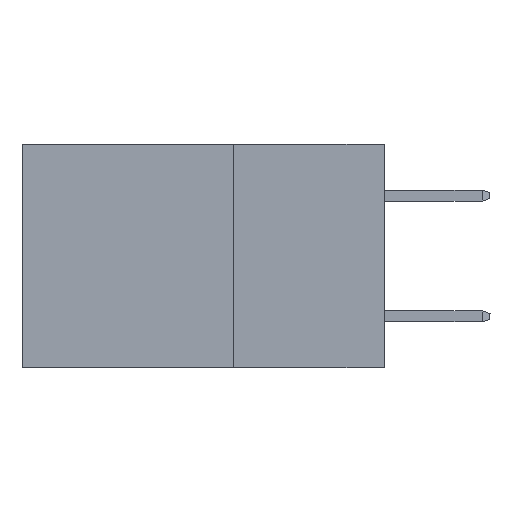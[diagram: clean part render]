
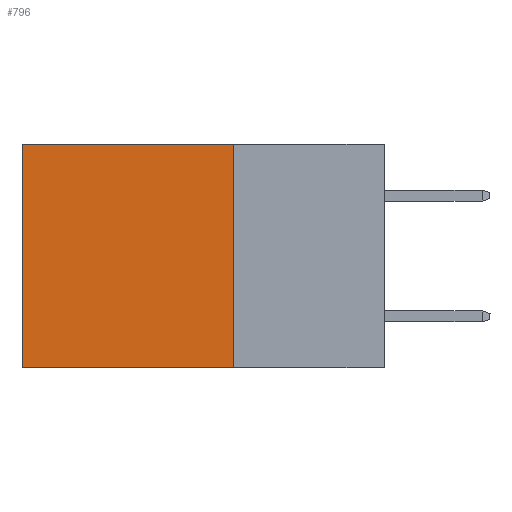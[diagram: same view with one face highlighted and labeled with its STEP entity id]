
A CAD part, left-side view. The second image highlights one B-rep face of the part: STEP entity #796.
In plain terms, the highlighted planar face has unit normal (-1, 0, 0).
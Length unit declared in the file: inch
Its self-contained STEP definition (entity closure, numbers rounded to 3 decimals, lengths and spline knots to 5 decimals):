
#796 = ADVANCED_FACE ( 'NONE', ( #2984 ), #13922, .F. ) ;
#869 = DIRECTION ( 'NONE',  ( 0., 0., -1. ) ) ;
#1543 = VECTOR ( 'NONE', #10704, 39.37008 ) ;
#2364 = LINE ( 'NONE', #10731, #1543 ) ;
#2478 = CARTESIAN_POINT ( 'NONE',  ( 0.2615, 0.6, -0.37 ) ) ;
#2984 = FACE_OUTER_BOUND ( 'NONE', #6601, .T. ) ;
#3396 = DIRECTION ( 'NONE',  ( 0., 1., 0. ) ) ;
#3472 = CARTESIAN_POINT ( 'NONE',  ( 0.2615, 0.25, 0. ) ) ;
#4384 = CARTESIAN_POINT ( 'NONE',  ( 0.2615, 0.25, -0.37 ) ) ;
#4527 = VECTOR ( 'NONE', #3396, 39.37008 ) ;
#5455 = CARTESIAN_POINT ( 'NONE',  ( 0.2615, 0.25, -0.37 ) ) ;
#6601 = EDGE_LOOP ( 'NONE', ( #13447, #7660, #10757, #11123 ) ) ;
#6797 = EDGE_CURVE ( 'NONE', #12698, #7142, #2364, .T. ) ;
#6958 = CARTESIAN_POINT ( 'NONE',  ( 0.2615, 0.25, -0.37 ) ) ;
#7142 = VERTEX_POINT ( 'NONE', #8756 ) ;
#7660 = ORIENTED_EDGE ( 'NONE', *, *, #6797, .F. ) ;
#7968 = EDGE_CURVE ( 'NONE', #12488, #13347, #10762, .T. ) ;
#8534 = CARTESIAN_POINT ( 'NONE',  ( 0.2615, 0.25, 0. ) ) ;
#8626 = VECTOR ( 'NONE', #11744, 39.37008 ) ;
#8756 = CARTESIAN_POINT ( 'NONE',  ( 0.2615, 0.6, -0.37 ) ) ;
#9367 = AXIS2_PLACEMENT_3D ( 'NONE', #4384, #14009, #14481 ) ;
#10704 = DIRECTION ( 'NONE',  ( 0., 1., 0. ) ) ;
#10731 = CARTESIAN_POINT ( 'NONE',  ( 0.2615, 0.25, -0.37 ) ) ;
#10757 = ORIENTED_EDGE ( 'NONE', *, *, #14665, .F. ) ;
#10762 = LINE ( 'NONE', #3472, #4527 ) ;
#11123 = ORIENTED_EDGE ( 'NONE', *, *, #7968, .T. ) ;
#11479 = LINE ( 'NONE', #6958, #14228 ) ;
#11744 = DIRECTION ( 'NONE',  ( 0., 0., -1. ) ) ;
#12488 = VERTEX_POINT ( 'NONE', #8534 ) ;
#12698 = VERTEX_POINT ( 'NONE', #5455 ) ;
#13315 = CARTESIAN_POINT ( 'NONE',  ( 0.2615, 0.6, 0. ) ) ;
#13347 = VERTEX_POINT ( 'NONE', #13315 ) ;
#13447 = ORIENTED_EDGE ( 'NONE', *, *, #14862, .T. ) ;
#13922 = PLANE ( 'NONE',  #9367 ) ;
#14009 = DIRECTION ( 'NONE',  ( 1., 0., 0. ) ) ;
#14228 = VECTOR ( 'NONE', #869, 39.37008 ) ;
#14481 = DIRECTION ( 'NONE',  ( 0., 0., -1. ) ) ;
#14665 = EDGE_CURVE ( 'NONE', #12488, #12698, #11479, .T. ) ;
#14715 = LINE ( 'NONE', #2478, #8626 ) ;
#14862 = EDGE_CURVE ( 'NONE', #13347, #7142, #14715, .T. ) ;
